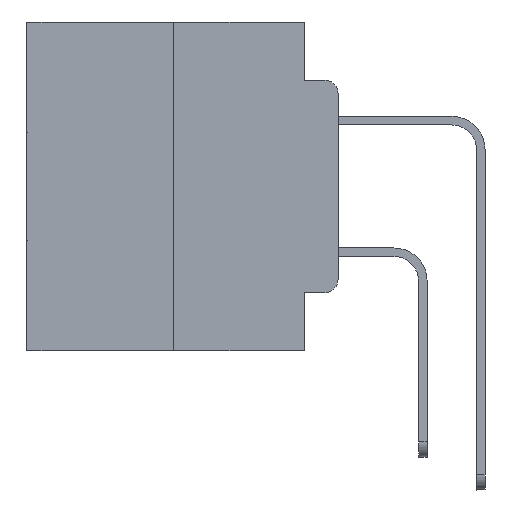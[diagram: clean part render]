
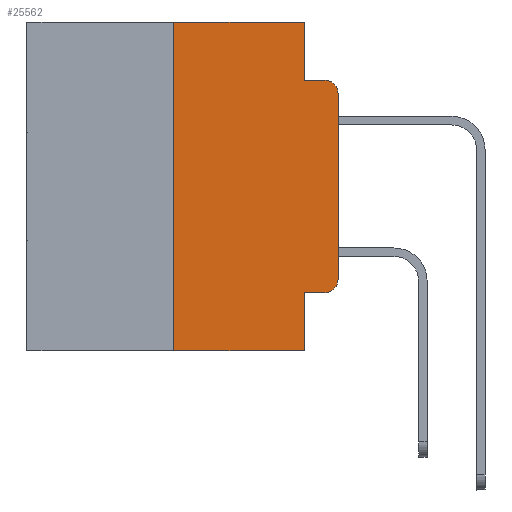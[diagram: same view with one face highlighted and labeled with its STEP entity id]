
A CAD part, left-side view. The second image highlights one B-rep face of the part: STEP entity #25562.
In plain terms, the highlighted planar face has unit normal (-1, 0, 0).
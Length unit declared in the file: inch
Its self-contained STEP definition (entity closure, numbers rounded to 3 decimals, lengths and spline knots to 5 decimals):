
#427 = LINE ( 'NONE', #17279, #25175 ) ;
#617 = CARTESIAN_POINT ( 'NONE',  ( 0., 0., -0.1085 ) ) ;
#848 = DIRECTION ( 'NONE',  ( 0., -1., 0. ) ) ;
#1808 = VECTOR ( 'NONE', #24296, 39.37008 ) ;
#2196 = VECTOR ( 'NONE', #27067, 39.37008 ) ;
#2531 = CARTESIAN_POINT ( 'NONE',  ( 0., 0.25, 0. ) ) ;
#2583 = CARTESIAN_POINT ( 'NONE',  ( 0., 0.051, 0. ) ) ;
#2695 = VECTOR ( 'NONE', #14886, 39.37008 ) ;
#3974 = EDGE_CURVE ( 'NONE', #24320, #16072, #19030, .T. ) ;
#4260 = CARTESIAN_POINT ( 'NONE',  ( 0., 0.02, -0.3915 ) ) ;
#4731 = VECTOR ( 'NONE', #16742, 39.37008 ) ;
#5818 = CARTESIAN_POINT ( 'NONE',  ( 0., 0.25, 0. ) ) ;
#6112 = EDGE_LOOP ( 'NONE', ( #7839, #8150, #8794, #9605, #9720, #9747, #10023, #10082, #10304, #10582 ) ) ;
#6644 = CARTESIAN_POINT ( 'NONE',  ( 0., 0.473, 0. ) ) ;
#6653 = DIRECTION ( 'NONE',  ( 0., 0., -1. ) ) ;
#6746 = EDGE_CURVE ( 'NONE', #28455, #29212, #18138, .T. ) ;
#7168 = CARTESIAN_POINT ( 'NONE',  ( 0., 0., 0. ) ) ;
#7621 = AXIS2_PLACEMENT_3D ( 'NONE', #26264, #12570, #28523 ) ;
#7839 = ORIENTED_EDGE ( 'NONE', *, *, #22288, .T. ) ;
#8150 = ORIENTED_EDGE ( 'NONE', *, *, #20755, .T. ) ;
#8340 = EDGE_CURVE ( 'NONE', #15861, #28455, #427, .T. ) ;
#8711 = VECTOR ( 'NONE', #9583, 39.37008 ) ;
#8794 = ORIENTED_EDGE ( 'NONE', *, *, #16126, .F. ) ;
#9183 = CARTESIAN_POINT ( 'NONE',  ( 0., 0.25, -0.5 ) ) ;
#9505 = VECTOR ( 'NONE', #23345, 39.37008 ) ;
#9583 = DIRECTION ( 'NONE',  ( 0., 0., 1. ) ) ;
#9605 = ORIENTED_EDGE ( 'NONE', *, *, #14569, .F. ) ;
#9720 = ORIENTED_EDGE ( 'NONE', *, *, #20795, .F. ) ;
#9742 = LINE ( 'NONE', #24107, #2695 ) ;
#9747 = ORIENTED_EDGE ( 'NONE', *, *, #13034, .F. ) ;
#10023 = ORIENTED_EDGE ( 'NONE', *, *, #3974, .T. ) ;
#10082 = ORIENTED_EDGE ( 'NONE', *, *, #11498, .F. ) ;
#10304 = ORIENTED_EDGE ( 'NONE', *, *, #8340, .T. ) ;
#10514 = AXIS2_PLACEMENT_3D ( 'NONE', #4260, #20554, #6653 ) ;
#10539 = CARTESIAN_POINT ( 'NONE',  ( 0., 0.473, -0.5 ) ) ;
#10582 = ORIENTED_EDGE ( 'NONE', *, *, #6746, .T. ) ;
#11167 = CARTESIAN_POINT ( 'NONE',  ( 0., 0., -0.3915 ) ) ;
#11397 = DIRECTION ( 'NONE',  ( 1., 0., 0. ) ) ;
#11498 = EDGE_CURVE ( 'NONE', #15861, #16072, #23960, .T. ) ;
#12000 = VERTEX_POINT ( 'NONE', #617 ) ;
#12570 = DIRECTION ( 'NONE',  ( -1., 0., 0. ) ) ;
#12866 = CARTESIAN_POINT ( 'NONE',  ( 0., 0.051, 0. ) ) ;
#13034 = EDGE_CURVE ( 'NONE', #24320, #27895, #14903, .T. ) ;
#13601 = PLANE ( 'NONE',  #14142 ) ;
#14142 = AXIS2_PLACEMENT_3D ( 'NONE', #6644, #11397, #27369 ) ;
#14569 = EDGE_CURVE ( 'NONE', #15035, #18742, #28001, .T. ) ;
#14711 = LINE ( 'NONE', #24818, #2196 ) ;
#14886 = DIRECTION ( 'NONE',  ( 0., -1., 0. ) ) ;
#14903 = LINE ( 'NONE', #2531, #8711 ) ;
#14952 = LINE ( 'NONE', #7168, #9505 ) ;
#15035 = VERTEX_POINT ( 'NONE', #23392 ) ;
#15191 = DIRECTION ( 'NONE',  ( 0., 0., -1. ) ) ;
#15861 = VERTEX_POINT ( 'NONE', #21753 ) ;
#15895 = VECTOR ( 'NONE', #15191, 39.37008 ) ;
#16072 = VERTEX_POINT ( 'NONE', #26883 ) ;
#16126 = EDGE_CURVE ( 'NONE', #18742, #17880, #14711, .T. ) ;
#16742 = DIRECTION ( 'NONE',  ( 0., 0., -1. ) ) ;
#17117 = CARTESIAN_POINT ( 'NONE',  ( 0., 0.02, -0.4115 ) ) ;
#17279 = CARTESIAN_POINT ( 'NONE',  ( 0., 0.051, -0.4115 ) ) ;
#17651 = CARTESIAN_POINT ( 'NONE',  ( 0., 0.051, -0.0885 ) ) ;
#17880 = VERTEX_POINT ( 'NONE', #19278 ) ;
#18138 = CIRCLE ( 'NONE', #10514, 0.02 ) ;
#18742 = VERTEX_POINT ( 'NONE', #17651 ) ;
#19030 = LINE ( 'NONE', #10539, #1808 ) ;
#19278 = CARTESIAN_POINT ( 'NONE',  ( 0., 0.02, -0.0885 ) ) ;
#20554 = DIRECTION ( 'NONE',  ( -1., 0., 0. ) ) ;
#20755 = EDGE_CURVE ( 'NONE', #12000, #17880, #22032, .T. ) ;
#20795 = EDGE_CURVE ( 'NONE', #27895, #15035, #9742, .T. ) ;
#21753 = CARTESIAN_POINT ( 'NONE',  ( 0., 0.051, -0.4115 ) ) ;
#22032 = CIRCLE ( 'NONE', #7621, 0.02 ) ;
#22288 = EDGE_CURVE ( 'NONE', #29212, #12000, #14952, .T. ) ;
#23345 = DIRECTION ( 'NONE',  ( 0., 0., 1. ) ) ;
#23392 = CARTESIAN_POINT ( 'NONE',  ( 0., 0.051, 0. ) ) ;
#23960 = LINE ( 'NONE', #2583, #4731 ) ;
#24107 = CARTESIAN_POINT ( 'NONE',  ( 0., 0.473, 0. ) ) ;
#24296 = DIRECTION ( 'NONE',  ( 0., -1., 0. ) ) ;
#24320 = VERTEX_POINT ( 'NONE', #9183 ) ;
#24818 = CARTESIAN_POINT ( 'NONE',  ( 0., 0.051, -0.0885 ) ) ;
#25175 = VECTOR ( 'NONE', #848, 39.37008 ) ;
#25562 = ADVANCED_FACE ( 'NONE', ( #27633 ), #13601, .F. ) ;
#26264 = CARTESIAN_POINT ( 'NONE',  ( 0., 0.02, -0.1085 ) ) ;
#26883 = CARTESIAN_POINT ( 'NONE',  ( 0., 0.051, -0.5 ) ) ;
#27067 = DIRECTION ( 'NONE',  ( 0., -1., 0. ) ) ;
#27369 = DIRECTION ( 'NONE',  ( 0., 0., -1. ) ) ;
#27633 = FACE_OUTER_BOUND ( 'NONE', #6112, .T. ) ;
#27895 = VERTEX_POINT ( 'NONE', #5818 ) ;
#28001 = LINE ( 'NONE', #12866, #15895 ) ;
#28455 = VERTEX_POINT ( 'NONE', #17117 ) ;
#28523 = DIRECTION ( 'NONE',  ( 0., 0., -1. ) ) ;
#29212 = VERTEX_POINT ( 'NONE', #11167 ) ;
